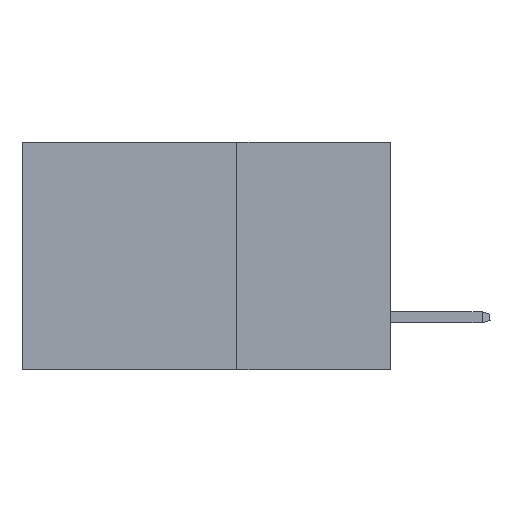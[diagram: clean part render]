
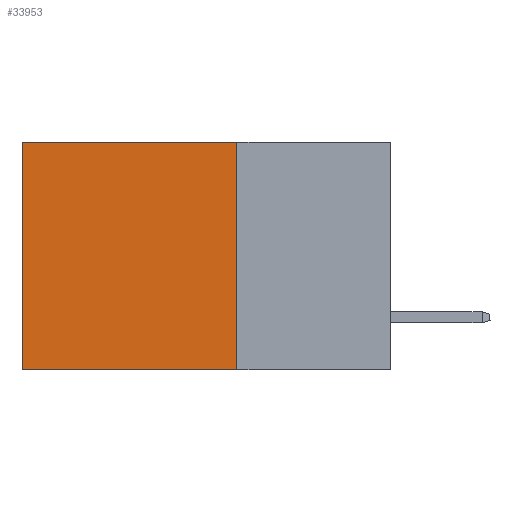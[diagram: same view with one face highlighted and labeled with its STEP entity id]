
A CAD part, left-side view. The second image highlights one B-rep face of the part: STEP entity #33953.
In plain terms, the highlighted planar face has unit normal (-1, 0, 0).
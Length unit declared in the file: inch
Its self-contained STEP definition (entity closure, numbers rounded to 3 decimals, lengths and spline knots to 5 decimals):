
#876 = CARTESIAN_POINT ( 'NONE',  ( 0.2875, 0.25, -0.37 ) ) ;
#1698 = VECTOR ( 'NONE', #30689, 39.37008 ) ;
#1747 = CARTESIAN_POINT ( 'NONE',  ( 0.2875, 0.25, -0.37 ) ) ;
#5465 = LINE ( 'NONE', #36126, #35604 ) ;
#6231 = DIRECTION ( 'NONE',  ( 0., 0., -1. ) ) ;
#8100 = CARTESIAN_POINT ( 'NONE',  ( 0.2875, 0.6, 0. ) ) ;
#8191 = LINE ( 'NONE', #8100, #1698 ) ;
#11962 = VERTEX_POINT ( 'NONE', #876 ) ;
#12210 = VECTOR ( 'NONE', #28460, 39.37008 ) ;
#13374 = LINE ( 'NONE', #1747, #44729 ) ;
#17519 = EDGE_CURVE ( 'NONE', #17912, #11962, #5465, .T. ) ;
#17912 = VERTEX_POINT ( 'NONE', #27654 ) ;
#20180 = VERTEX_POINT ( 'NONE', #31299 ) ;
#20365 = ORIENTED_EDGE ( 'NONE', *, *, #21418, .T. ) ;
#21418 = EDGE_CURVE ( 'NONE', #17912, #20180, #47650, .T. ) ;
#21489 = EDGE_CURVE ( 'NONE', #11962, #28680, #13374, .T. ) ;
#24123 = ORIENTED_EDGE ( 'NONE', *, *, #21489, .F. ) ;
#24657 = AXIS2_PLACEMENT_3D ( 'NONE', #47235, #47572, #24906 ) ;
#24906 = DIRECTION ( 'NONE',  ( 0., 0., -1. ) ) ;
#26515 = CARTESIAN_POINT ( 'NONE',  ( 0.2875, 0.6, -0.37 ) ) ;
#27654 = CARTESIAN_POINT ( 'NONE',  ( 0.2875, 0.25, 0. ) ) ;
#28460 = DIRECTION ( 'NONE',  ( 0., 1., 0. ) ) ;
#28680 = VERTEX_POINT ( 'NONE', #26515 ) ;
#30689 = DIRECTION ( 'NONE',  ( 0., 0., -1. ) ) ;
#31299 = CARTESIAN_POINT ( 'NONE',  ( 0.2875, 0.6, 0. ) ) ;
#33232 = ORIENTED_EDGE ( 'NONE', *, *, #38392, .T. ) ;
#33953 = ADVANCED_FACE ( 'NONE', ( #44138 ), #43470, .F. ) ;
#35604 = VECTOR ( 'NONE', #6231, 39.37008 ) ;
#36126 = CARTESIAN_POINT ( 'NONE',  ( 0.2875, 0.25, 0. ) ) ;
#38392 = EDGE_CURVE ( 'NONE', #20180, #28680, #8191, .T. ) ;
#39383 = CARTESIAN_POINT ( 'NONE',  ( 0.2875, 0.25, 0. ) ) ;
#39717 = DIRECTION ( 'NONE',  ( 0., 1., 0. ) ) ;
#43470 = PLANE ( 'NONE',  #24657 ) ;
#44138 = FACE_OUTER_BOUND ( 'NONE', #44326, .T. ) ;
#44326 = EDGE_LOOP ( 'NONE', ( #33232, #24123, #44805, #20365 ) ) ;
#44729 = VECTOR ( 'NONE', #39717, 39.37008 ) ;
#44805 = ORIENTED_EDGE ( 'NONE', *, *, #17519, .F. ) ;
#47235 = CARTESIAN_POINT ( 'NONE',  ( 0.2875, 0.25, 0. ) ) ;
#47572 = DIRECTION ( 'NONE',  ( 1., 0., 0. ) ) ;
#47650 = LINE ( 'NONE', #39383, #12210 ) ;
